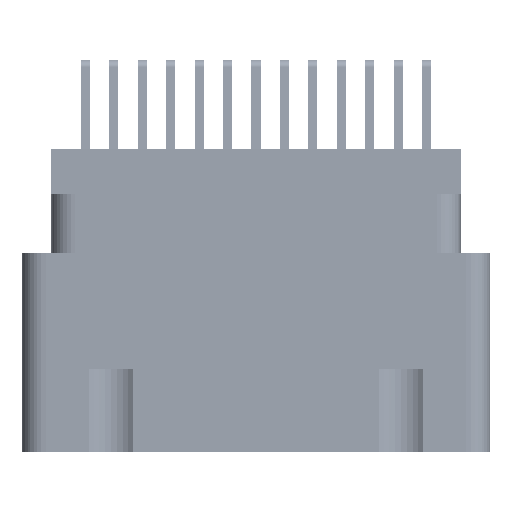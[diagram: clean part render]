
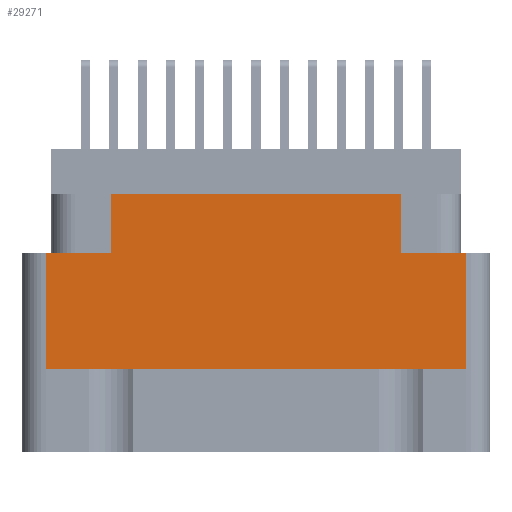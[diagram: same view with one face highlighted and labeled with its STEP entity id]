
A CAD part, left-side view. The second image highlights one B-rep face of the part: STEP entity #29271.
In plain terms, the highlighted planar face has unit normal (-1, 0, 0).
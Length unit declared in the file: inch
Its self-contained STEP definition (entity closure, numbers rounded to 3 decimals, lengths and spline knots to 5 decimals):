
#61 = VECTOR ( 'NONE', #15345, 39.37008 ) ;
#1036 = CARTESIAN_POINT ( 'NONE',  ( -1.359, 0.3825, -0.117 ) ) ;
#1462 = CARTESIAN_POINT ( 'NONE',  ( -1.359, -0.555, -0.578 ) ) ;
#1828 = LINE ( 'NONE', #4187, #61 ) ;
#1879 = ORIENTED_EDGE ( 'NONE', *, *, #5286, .F. ) ;
#1909 = LINE ( 'NONE', #12830, #26159 ) ;
#2385 = EDGE_CURVE ( 'NONE', #12062, #4796, #50420, .T. ) ;
#2637 = LINE ( 'NONE', #50422, #26036 ) ;
#2732 = LINE ( 'NONE', #13544, #60710 ) ;
#3384 = PLANE ( 'NONE',  #69590 ) ;
#4187 = CARTESIAN_POINT ( 'NONE',  ( -1.359, 0.3825, -0.274 ) ) ;
#4556 = EDGE_CURVE ( 'NONE', #4796, #68375, #1828, .T. ) ;
#4796 = VERTEX_POINT ( 'NONE', #53737 ) ;
#5005 = ORIENTED_EDGE ( 'NONE', *, *, #2385, .F. ) ;
#5286 = EDGE_CURVE ( 'NONE', #62703, #67113, #2732, .T. ) ;
#7083 = EDGE_CURVE ( 'NONE', #36845, #67113, #48900, .T. ) ;
#8520 = LINE ( 'NONE', #10795, #37981 ) ;
#10795 = CARTESIAN_POINT ( 'NONE',  ( -1.359, -0.3825, -0.274 ) ) ;
#11118 = CARTESIAN_POINT ( 'NONE',  ( -1.359, -0.555, -0.274 ) ) ;
#11147 = DIRECTION ( 'NONE',  ( 0., -1., 0. ) ) ;
#11258 = EDGE_CURVE ( 'NONE', #68375, #23598, #69114, .T. ) ;
#12062 = VERTEX_POINT ( 'NONE', #27533 ) ;
#12830 = CARTESIAN_POINT ( 'NONE',  ( -1.359, 0., -0.578 ) ) ;
#13544 = CARTESIAN_POINT ( 'NONE',  ( -1.359, 0., -0.274 ) ) ;
#15345 = DIRECTION ( 'NONE',  ( 0., 0., 1. ) ) ;
#17270 = DIRECTION ( 'NONE',  ( 0., 0., -1. ) ) ;
#18040 = ORIENTED_EDGE ( 'NONE', *, *, #7083, .T. ) ;
#18382 = DIRECTION ( 'NONE',  ( 0., -1., 0. ) ) ;
#18831 = CARTESIAN_POINT ( 'NONE',  ( -1.359, -0.3825, -0.274 ) ) ;
#19428 = VECTOR ( 'NONE', #22798, 39.37008 ) ;
#19457 = CARTESIAN_POINT ( 'NONE',  ( -1.359, 0.555, -0.578 ) ) ;
#21171 = VERTEX_POINT ( 'NONE', #19457 ) ;
#22798 = DIRECTION ( 'NONE',  ( 0., 0., 1. ) ) ;
#23598 = VERTEX_POINT ( 'NONE', #45436 ) ;
#24471 = DIRECTION ( 'NONE',  ( 0., 0., 1. ) ) ;
#26036 = VECTOR ( 'NONE', #17270, 39.37008 ) ;
#26159 = VECTOR ( 'NONE', #18382, 39.37008 ) ;
#26673 = CARTESIAN_POINT ( 'NONE',  ( -1.359, 0.617, -0.117 ) ) ;
#27135 = ORIENTED_EDGE ( 'NONE', *, *, #33692, .T. ) ;
#27533 = CARTESIAN_POINT ( 'NONE',  ( -1.359, 0.555, -0.274 ) ) ;
#29271 = ADVANCED_FACE ( 'NONE', ( #59138 ), #3384, .T. ) ;
#32373 = DIRECTION ( 'NONE',  ( 0., 0., 1. ) ) ;
#33023 = ORIENTED_EDGE ( 'NONE', *, *, #65662, .T. ) ;
#33048 = DIRECTION ( 'NONE',  ( 0., -1., 0. ) ) ;
#33692 = EDGE_CURVE ( 'NONE', #12062, #21171, #2637, .T. ) ;
#34850 = CARTESIAN_POINT ( 'NONE',  ( -1.359, -0.555, -0.798 ) ) ;
#36845 = VERTEX_POINT ( 'NONE', #1462 ) ;
#37904 = CARTESIAN_POINT ( 'NONE',  ( -1.359, 0., -0.274 ) ) ;
#37981 = VECTOR ( 'NONE', #32373, 39.37008 ) ;
#41315 = EDGE_CURVE ( 'NONE', #21171, #36845, #1909, .T. ) ;
#42423 = ORIENTED_EDGE ( 'NONE', *, *, #11258, .F. ) ;
#43805 = ORIENTED_EDGE ( 'NONE', *, *, #41315, .T. ) ;
#45436 = CARTESIAN_POINT ( 'NONE',  ( -1.359, -0.3825, -0.117 ) ) ;
#47008 = DIRECTION ( 'NONE',  ( -1., 0., 0. ) ) ;
#47241 = DIRECTION ( 'NONE',  ( 0., -1., 0. ) ) ;
#47713 = CARTESIAN_POINT ( 'NONE',  ( -1.359, -0.617, -0.798 ) ) ;
#48900 = LINE ( 'NONE', #34850, #19428 ) ;
#50420 = LINE ( 'NONE', #37904, #54764 ) ;
#50422 = CARTESIAN_POINT ( 'NONE',  ( -1.359, 0.555, -0.798 ) ) ;
#53737 = CARTESIAN_POINT ( 'NONE',  ( -1.359, 0.3825, -0.274 ) ) ;
#54502 = VECTOR ( 'NONE', #11147, 39.37008 ) ;
#54764 = VECTOR ( 'NONE', #33048, 39.37008 ) ;
#56282 = ORIENTED_EDGE ( 'NONE', *, *, #4556, .F. ) ;
#57519 = EDGE_LOOP ( 'NONE', ( #5005, #27135, #43805, #18040, #1879, #33023, #42423, #56282 ) ) ;
#59138 = FACE_OUTER_BOUND ( 'NONE', #57519, .T. ) ;
#60710 = VECTOR ( 'NONE', #47241, 39.37008 ) ;
#62703 = VERTEX_POINT ( 'NONE', #18831 ) ;
#65662 = EDGE_CURVE ( 'NONE', #62703, #23598, #8520, .T. ) ;
#67113 = VERTEX_POINT ( 'NONE', #11118 ) ;
#68375 = VERTEX_POINT ( 'NONE', #1036 ) ;
#69114 = LINE ( 'NONE', #26673, #54502 ) ;
#69590 = AXIS2_PLACEMENT_3D ( 'NONE', #47713, #47008, #24471 ) ;
